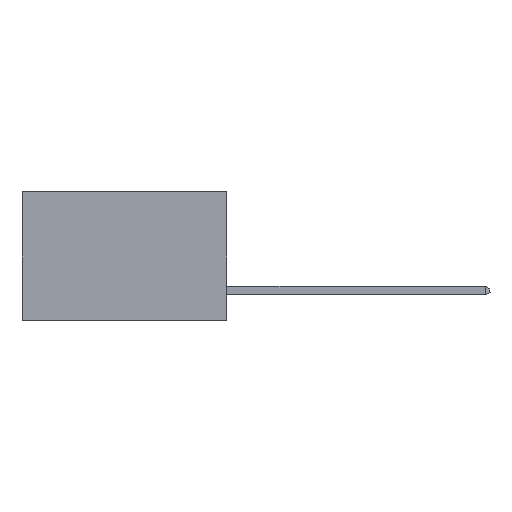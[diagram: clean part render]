
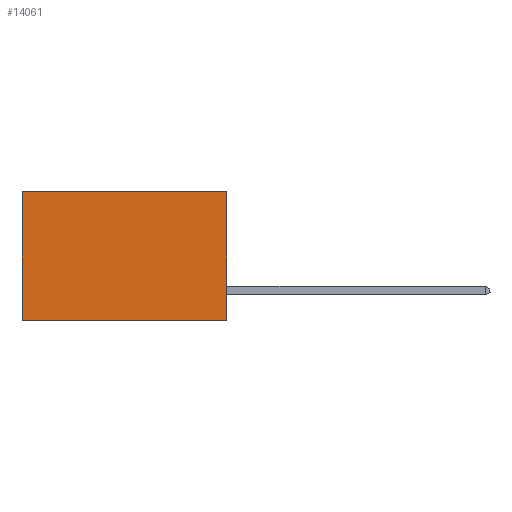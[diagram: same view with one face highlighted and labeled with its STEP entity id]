
A CAD part, left-side view. The second image highlights one B-rep face of the part: STEP entity #14061.
In plain terms, the highlighted planar face has unit normal (-1, 0, 0).
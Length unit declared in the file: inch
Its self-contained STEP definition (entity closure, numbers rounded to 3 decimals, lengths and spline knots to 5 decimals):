
#957 = VERTEX_POINT ( 'NONE', #4492 ) ;
#1197 = VECTOR ( 'NONE', #2327, 39.37008 ) ;
#2327 = DIRECTION ( 'NONE',  ( 0., 0., -1. ) ) ;
#3819 = VERTEX_POINT ( 'NONE', #16379 ) ;
#4188 = LINE ( 'NONE', #9999, #15325 ) ;
#4492 = CARTESIAN_POINT ( 'NONE',  ( 0.277, 0., -0.37 ) ) ;
#5167 = DIRECTION ( 'NONE',  ( 0., 1., 0. ) ) ;
#5458 = CARTESIAN_POINT ( 'NONE',  ( 0.277, 0., -0.37 ) ) ;
#6196 = ORIENTED_EDGE ( 'NONE', *, *, #12456, .T. ) ;
#6768 = EDGE_LOOP ( 'NONE', ( #7063, #19212, #8690, #6196 ) ) ;
#6856 = CARTESIAN_POINT ( 'NONE',  ( 0.277, 0.59, -0.37 ) ) ;
#6868 = EDGE_CURVE ( 'NONE', #957, #9856, #15253, .T. ) ;
#6971 = VECTOR ( 'NONE', #12034, 39.37008 ) ;
#6999 = CARTESIAN_POINT ( 'NONE',  ( 0.277, 0., 0. ) ) ;
#7063 = ORIENTED_EDGE ( 'NONE', *, *, #16170, .T. ) ;
#8690 = ORIENTED_EDGE ( 'NONE', *, *, #14026, .F. ) ;
#9856 = VERTEX_POINT ( 'NONE', #14692 ) ;
#9999 = CARTESIAN_POINT ( 'NONE',  ( 0.277, 0., 0. ) ) ;
#10108 = DIRECTION ( 'NONE',  ( 0., 1., 0. ) ) ;
#10299 = CARTESIAN_POINT ( 'NONE',  ( 0.277, 0., -0.37 ) ) ;
#10394 = VERTEX_POINT ( 'NONE', #6999 ) ;
#10524 = FACE_OUTER_BOUND ( 'NONE', #6768, .T. ) ;
#10844 = DIRECTION ( 'NONE',  ( 0., 0., -1. ) ) ;
#10922 = DIRECTION ( 'NONE',  ( 1., 0., 0. ) ) ;
#10960 = CARTESIAN_POINT ( 'NONE',  ( 0.277, 0., -0.37 ) ) ;
#11089 = PLANE ( 'NONE',  #12633 ) ;
#12034 = DIRECTION ( 'NONE',  ( 0., 0., -1. ) ) ;
#12456 = EDGE_CURVE ( 'NONE', #10394, #3819, #4188, .T. ) ;
#12633 = AXIS2_PLACEMENT_3D ( 'NONE', #10960, #10922, #10844 ) ;
#13267 = LINE ( 'NONE', #6856, #1197 ) ;
#14026 = EDGE_CURVE ( 'NONE', #10394, #957, #18888, .T. ) ;
#14061 = ADVANCED_FACE ( 'NONE', ( #10524 ), #11089, .F. ) ;
#14311 = VECTOR ( 'NONE', #5167, 39.37008 ) ;
#14692 = CARTESIAN_POINT ( 'NONE',  ( 0.277, 0.59, -0.37 ) ) ;
#15253 = LINE ( 'NONE', #5458, #14311 ) ;
#15325 = VECTOR ( 'NONE', #10108, 39.37008 ) ;
#16170 = EDGE_CURVE ( 'NONE', #3819, #9856, #13267, .T. ) ;
#16379 = CARTESIAN_POINT ( 'NONE',  ( 0.277, 0.59, 0. ) ) ;
#18888 = LINE ( 'NONE', #10299, #6971 ) ;
#19212 = ORIENTED_EDGE ( 'NONE', *, *, #6868, .F. ) ;
